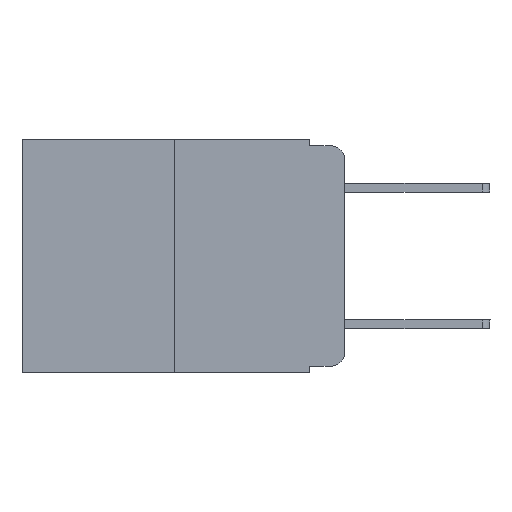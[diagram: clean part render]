
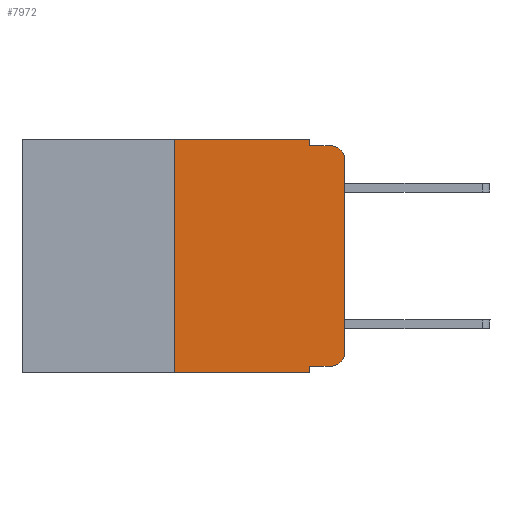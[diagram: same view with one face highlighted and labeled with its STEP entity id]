
A CAD part, left-side view. The second image highlights one B-rep face of the part: STEP entity #7972.
In plain terms, the highlighted planar face has unit normal (-1, 0, 0).
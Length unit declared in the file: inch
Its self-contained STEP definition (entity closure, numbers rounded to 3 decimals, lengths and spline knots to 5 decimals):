
#590 = LINE ( 'NONE', #13928, #17398 ) ;
#703 = AXIS2_PLACEMENT_3D ( 'NONE', #17438, #12455, #15910 ) ;
#1011 = DIRECTION ( 'NONE',  ( 0., 0., -1. ) ) ;
#1217 = VECTOR ( 'NONE', #16917, 39.37008 ) ;
#1328 = ORIENTED_EDGE ( 'NONE', *, *, #13747, .F. ) ;
#1332 = CARTESIAN_POINT ( 'NONE',  ( 0., 0.051, -0.333 ) ) ;
#1531 = LINE ( 'NONE', #8093, #9235 ) ;
#1976 = EDGE_CURVE ( 'NONE', #20294, #9857, #7431, .T. ) ;
#2013 = CARTESIAN_POINT ( 'NONE',  ( 0., 0., 0. ) ) ;
#2301 = DIRECTION ( 'NONE',  ( 0., 0., -1. ) ) ;
#2403 = LINE ( 'NONE', #8745, #7454 ) ;
#2701 = EDGE_CURVE ( 'NONE', #16816, #8919, #6621, .T. ) ;
#3215 = EDGE_CURVE ( 'NONE', #12120, #15461, #2403, .T. ) ;
#3454 = CARTESIAN_POINT ( 'NONE',  ( 0., 0.473, 0. ) ) ;
#3824 = ORIENTED_EDGE ( 'NONE', *, *, #15208, .T. ) ;
#4127 = CARTESIAN_POINT ( 'NONE',  ( 0., 0.02, -0.03 ) ) ;
#4311 = CARTESIAN_POINT ( 'NONE',  ( 0., 0.051, 0. ) ) ;
#4829 = VECTOR ( 'NONE', #18112, 39.37008 ) ;
#5165 = CIRCLE ( 'NONE', #703, 0.02 ) ;
#5239 = DIRECTION ( 'NONE',  ( 0., 0., 1. ) ) ;
#5664 = VECTOR ( 'NONE', #16047, 39.37008 ) ;
#5704 = CARTESIAN_POINT ( 'NONE',  ( 0., 0.051, 0. ) ) ;
#5953 = EDGE_CURVE ( 'NONE', #17616, #16816, #8781, .T. ) ;
#6305 = AXIS2_PLACEMENT_3D ( 'NONE', #12630, #15981, #1011 ) ;
#6621 = CIRCLE ( 'NONE', #12131, 0.02 ) ;
#7351 = DIRECTION ( 'NONE',  ( 0., 0., 1. ) ) ;
#7431 = LINE ( 'NONE', #15941, #5664 ) ;
#7454 = VECTOR ( 'NONE', #7351, 39.37008 ) ;
#7587 = ORIENTED_EDGE ( 'NONE', *, *, #18846, .T. ) ;
#7642 = CARTESIAN_POINT ( 'NONE',  ( 0., 0.051, -0.01 ) ) ;
#7900 = ORIENTED_EDGE ( 'NONE', *, *, #1976, .F. ) ;
#7972 = ADVANCED_FACE ( 'NONE', ( #10381 ), #16967, .F. ) ;
#8058 = ORIENTED_EDGE ( 'NONE', *, *, #16685, .F. ) ;
#8093 = CARTESIAN_POINT ( 'NONE',  ( 0., 0.473, -0.343 ) ) ;
#8643 = DIRECTION ( 'NONE',  ( 0., -1., 0. ) ) ;
#8745 = CARTESIAN_POINT ( 'NONE',  ( 0., 0.25, 0. ) ) ;
#8781 = LINE ( 'NONE', #2013, #9814 ) ;
#8868 = VERTEX_POINT ( 'NONE', #4311 ) ;
#8919 = VERTEX_POINT ( 'NONE', #17352 ) ;
#9235 = VECTOR ( 'NONE', #14663, 39.37008 ) ;
#9814 = VECTOR ( 'NONE', #5239, 39.37008 ) ;
#9857 = VERTEX_POINT ( 'NONE', #16486 ) ;
#10005 = EDGE_CURVE ( 'NONE', #8868, #18356, #13668, .T. ) ;
#10381 = FACE_OUTER_BOUND ( 'NONE', #13456, .T. ) ;
#11925 = EDGE_CURVE ( 'NONE', #20294, #13213, #590, .T. ) ;
#12120 = VERTEX_POINT ( 'NONE', #15752 ) ;
#12131 = AXIS2_PLACEMENT_3D ( 'NONE', #4127, #17070, #2301 ) ;
#12370 = ORIENTED_EDGE ( 'NONE', *, *, #3215, .F. ) ;
#12455 = DIRECTION ( 'NONE',  ( -1., 0., 0. ) ) ;
#12630 = CARTESIAN_POINT ( 'NONE',  ( 0., 0.473, 0. ) ) ;
#13213 = VERTEX_POINT ( 'NONE', #18890 ) ;
#13456 = EDGE_LOOP ( 'NONE', ( #16761, #18263, #1328, #20941, #8058, #12370, #3824, #7900, #15304, #7587 ) ) ;
#13668 = LINE ( 'NONE', #5704, #1217 ) ;
#13747 = EDGE_CURVE ( 'NONE', #18356, #8919, #20151, .T. ) ;
#13928 = CARTESIAN_POINT ( 'NONE',  ( 0., 0.051, -0.333 ) ) ;
#14017 = VECTOR ( 'NONE', #20569, 39.37008 ) ;
#14503 = CARTESIAN_POINT ( 'NONE',  ( 0., 0., -0.313 ) ) ;
#14663 = DIRECTION ( 'NONE',  ( 0., -1., 0. ) ) ;
#15208 = EDGE_CURVE ( 'NONE', #12120, #9857, #1531, .T. ) ;
#15304 = ORIENTED_EDGE ( 'NONE', *, *, #11925, .T. ) ;
#15461 = VERTEX_POINT ( 'NONE', #17893 ) ;
#15752 = CARTESIAN_POINT ( 'NONE',  ( 0., 0.25, -0.343 ) ) ;
#15910 = DIRECTION ( 'NONE',  ( 0., 0., -1. ) ) ;
#15941 = CARTESIAN_POINT ( 'NONE',  ( 0., 0.051, 0. ) ) ;
#15981 = DIRECTION ( 'NONE',  ( 1., 0., 0. ) ) ;
#16047 = DIRECTION ( 'NONE',  ( 0., 0., -1. ) ) ;
#16486 = CARTESIAN_POINT ( 'NONE',  ( 0., 0.051, -0.343 ) ) ;
#16685 = EDGE_CURVE ( 'NONE', #15461, #8868, #17796, .T. ) ;
#16761 = ORIENTED_EDGE ( 'NONE', *, *, #5953, .T. ) ;
#16816 = VERTEX_POINT ( 'NONE', #18525 ) ;
#16917 = DIRECTION ( 'NONE',  ( 0., 0., -1. ) ) ;
#16967 = PLANE ( 'NONE',  #6305 ) ;
#17070 = DIRECTION ( 'NONE',  ( -1., 0., 0. ) ) ;
#17352 = CARTESIAN_POINT ( 'NONE',  ( 0., 0.02, -0.01 ) ) ;
#17398 = VECTOR ( 'NONE', #8643, 39.37008 ) ;
#17438 = CARTESIAN_POINT ( 'NONE',  ( 0., 0.02, -0.313 ) ) ;
#17616 = VERTEX_POINT ( 'NONE', #14503 ) ;
#17796 = LINE ( 'NONE', #3454, #4829 ) ;
#17893 = CARTESIAN_POINT ( 'NONE',  ( 0., 0.25, 0. ) ) ;
#18112 = DIRECTION ( 'NONE',  ( 0., -1., 0. ) ) ;
#18263 = ORIENTED_EDGE ( 'NONE', *, *, #2701, .T. ) ;
#18356 = VERTEX_POINT ( 'NONE', #7642 ) ;
#18525 = CARTESIAN_POINT ( 'NONE',  ( 0., 0., -0.03 ) ) ;
#18846 = EDGE_CURVE ( 'NONE', #13213, #17616, #5165, .T. ) ;
#18890 = CARTESIAN_POINT ( 'NONE',  ( 0., 0.02, -0.333 ) ) ;
#20151 = LINE ( 'NONE', #20358, #14017 ) ;
#20294 = VERTEX_POINT ( 'NONE', #1332 ) ;
#20358 = CARTESIAN_POINT ( 'NONE',  ( 0., 0.051, -0.01 ) ) ;
#20569 = DIRECTION ( 'NONE',  ( 0., -1., 0. ) ) ;
#20941 = ORIENTED_EDGE ( 'NONE', *, *, #10005, .F. ) ;
